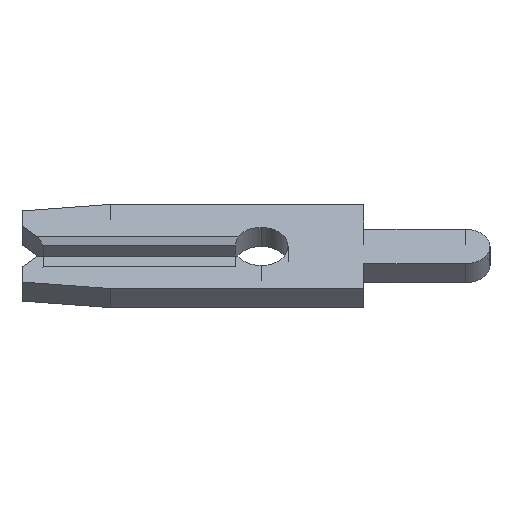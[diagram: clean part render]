
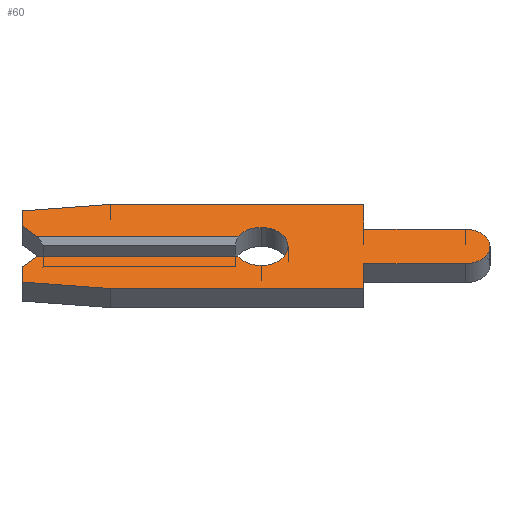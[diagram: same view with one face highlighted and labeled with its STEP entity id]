
A CAD part, left-side view. The second image highlights one B-rep face of the part: STEP entity #60.
In plain terms, the highlighted face is planar.
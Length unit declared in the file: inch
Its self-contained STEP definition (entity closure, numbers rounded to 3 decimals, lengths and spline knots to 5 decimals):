
#1 = LINE ( 'NONE', #1700, #1243 ) ;
#35 = DIRECTION ( 'NONE',  ( -1., 0., 0. ) ) ;
#55 = VECTOR ( 'NONE', #1398, 39.37008 ) ;
#60 = ADVANCED_FACE ( 'NONE', ( #71 ), #1540, .F. ) ;
#71 = FACE_OUTER_BOUND ( 'NONE', #1088, .T. ) ;
#76 = ORIENTED_EDGE ( 'NONE', *, *, #198, .F. ) ;
#86 = VECTOR ( 'NONE', #1055, 39.37008 ) ;
#87 = CARTESIAN_POINT ( 'NONE',  ( -0.013, -0.1975, -0.0235 ) ) ;
#91 = CARTESIAN_POINT ( 'NONE',  ( -0.013, -0.099, 0.0235 ) ) ;
#116 = EDGE_CURVE ( 'NONE', #1022, #850, #2049, .T. ) ;
#178 = VECTOR ( 'NONE', #1455, 39.37008 ) ;
#198 = EDGE_CURVE ( 'NONE', #300, #1527, #1787, .T. ) ;
#211 = ORIENTED_EDGE ( 'NONE', *, *, #1253, .F. ) ;
#213 = LINE ( 'NONE', #1473, #530 ) ;
#223 = VECTOR ( 'NONE', #612, 39.37008 ) ;
#226 = ORIENTED_EDGE ( 'NONE', *, *, #782, .F. ) ;
#241 = VECTOR ( 'NONE', #2071, 39.37008 ) ;
#256 = ORIENTED_EDGE ( 'NONE', *, *, #1232, .F. ) ;
#262 = CARTESIAN_POINT ( 'NONE',  ( -0.013, 0.146, -0.0575 ) ) ;
#300 = VERTEX_POINT ( 'NONE', #1580 ) ;
#330 = CARTESIAN_POINT ( 'NONE',  ( -0.013, 0.216, 0.013 ) ) ;
#331 = CARTESIAN_POINT ( 'NONE',  ( -0.013, -0.099, -0.0575 ) ) ;
#364 = DIRECTION ( 'NONE',  ( 0., 0., -1. ) ) ;
#389 = CARTESIAN_POINT ( 'NONE',  ( -0.013, 0.231, -0.028 ) ) ;
#399 = DIRECTION ( 'NONE',  ( 0., 0., -1. ) ) ;
#404 = ORIENTED_EDGE ( 'NONE', *, *, #1891, .F. ) ;
#419 = EDGE_CURVE ( 'NONE', #2013, #1078, #914, .T. ) ;
#432 = DIRECTION ( 'NONE',  ( 0., -1., 0. ) ) ;
#486 = ORIENTED_EDGE ( 'NONE', *, *, #760, .F. ) ;
#488 = ORIENTED_EDGE ( 'NONE', *, *, #1707, .F. ) ;
#492 = EDGE_CURVE ( 'NONE', #1858, #2013, #1421, .T. ) ;
#506 = LINE ( 'NONE', #1623, #223 ) ;
#515 = VERTEX_POINT ( 'NONE', #1100 ) ;
#530 = VECTOR ( 'NONE', #2150, 39.37008 ) ;
#537 = LINE ( 'NONE', #1904, #86 ) ;
#541 = ORIENTED_EDGE ( 'NONE', *, *, #1596, .F. ) ;
#547 = VERTEX_POINT ( 'NONE', #87 ) ;
#550 = VECTOR ( 'NONE', #1378, 39.37008 ) ;
#557 = VERTEX_POINT ( 'NONE', #590 ) ;
#568 = CARTESIAN_POINT ( 'NONE',  ( -0.013, 0.231, -0.04857 ) ) ;
#590 = CARTESIAN_POINT ( 'NONE',  ( -0.013, -0.099, 0.0235 ) ) ;
#593 = VERTEX_POINT ( 'NONE', #262 ) ;
#599 = CARTESIAN_POINT ( 'NONE',  ( -0.013, 0.146, 0.0575 ) ) ;
#612 = DIRECTION ( 'NONE',  ( 0., 1., 0. ) ) ;
#653 = DIRECTION ( 'NONE',  ( 1., 0., 0. ) ) ;
#684 = CARTESIAN_POINT ( 'NONE',  ( -0.013, 0.02252, 0.013 ) ) ;
#706 = DIRECTION ( 'NONE',  ( 1., 0., 0. ) ) ;
#720 = CARTESIAN_POINT ( 'NONE',  ( -0.013, -0.099, 0.0575 ) ) ;
#723 = LINE ( 'NONE', #1014, #1959 ) ;
#760 = EDGE_CURVE ( 'NONE', #1499, #2072, #213, .T. ) ;
#764 = CIRCLE ( 'NONE', #1404, 0.0235 ) ;
#771 = CARTESIAN_POINT ( 'NONE',  ( -0.013, 0., 0. ) ) ;
#782 = EDGE_CURVE ( 'NONE', #1078, #557, #1586, .T. ) ;
#793 = CIRCLE ( 'NONE', #1589, 0.026 ) ;
#801 = LINE ( 'NONE', #389, #1654 ) ;
#828 = DIRECTION ( 'NONE',  ( 0., 0.995, 0.105 ) ) ;
#840 = CARTESIAN_POINT ( 'NONE',  ( -0.013, 0.231, 0.028 ) ) ;
#844 = CARTESIAN_POINT ( 'NONE',  ( -0.013, 0.231, 0.04857 ) ) ;
#850 = VERTEX_POINT ( 'NONE', #1493 ) ;
#878 = DIRECTION ( 'NONE',  ( 0., 0., -1. ) ) ;
#879 = DIRECTION ( 'NONE',  ( 0., 1., 0. ) ) ;
#898 = DIRECTION ( 'NONE',  ( 0., 0., 1. ) ) ;
#910 = DIRECTION ( 'NONE',  ( 0., -1., 0. ) ) ;
#914 = LINE ( 'NONE', #599, #1304 ) ;
#919 = CARTESIAN_POINT ( 'NONE',  ( -0.013, 0., 0.026 ) ) ;
#953 = ORIENTED_EDGE ( 'NONE', *, *, #2076, .F. ) ;
#975 = EDGE_CURVE ( 'NONE', #515, #547, #764, .T. ) ;
#996 = CARTESIAN_POINT ( 'NONE',  ( -0.013, 0.02252, -0.013 ) ) ;
#1001 = EDGE_CURVE ( 'NONE', #2052, #300, #1039, .T. ) ;
#1014 = CARTESIAN_POINT ( 'NONE',  ( -0.013, 0.231, -0.04857 ) ) ;
#1022 = VERTEX_POINT ( 'NONE', #330 ) ;
#1039 = CIRCLE ( 'NONE', #1171, 0.026 ) ;
#1055 = DIRECTION ( 'NONE',  ( 0., -1., 0. ) ) ;
#1078 = VERTEX_POINT ( 'NONE', #2054 ) ;
#1088 = EDGE_LOOP ( 'NONE', ( #1475, #1601, #76, #2011, #2145, #211, #2048, #404, #953, #486, #488, #1652, #541, #226, #1982, #2135, #256, #1816 ) ) ;
#1100 = CARTESIAN_POINT ( 'NONE',  ( -0.013, -0.1975, 0.0235 ) ) ;
#1106 = LINE ( 'NONE', #1157, #1890 ) ;
#1121 = LINE ( 'NONE', #91, #1343 ) ;
#1136 = LINE ( 'NONE', #840, #55 ) ;
#1147 = CARTESIAN_POINT ( 'NONE',  ( -0.013, 0.231, -0.028 ) ) ;
#1157 = CARTESIAN_POINT ( 'NONE',  ( -0.013, 0.146, -0.0575 ) ) ;
#1164 = DIRECTION ( 'NONE',  ( 0., -1., 0. ) ) ;
#1171 = AXIS2_PLACEMENT_3D ( 'NONE', #2062, #35, #878 ) ;
#1186 = VERTEX_POINT ( 'NONE', #684 ) ;
#1196 = CARTESIAN_POINT ( 'NONE',  ( -0.013, 0.2105, 0.0075 ) ) ;
#1214 = DIRECTION ( 'NONE',  ( 0., -0.707, 0.707 ) ) ;
#1232 = EDGE_CURVE ( 'NONE', #850, #1858, #1136, .T. ) ;
#1243 = VECTOR ( 'NONE', #1164, 39.37008 ) ;
#1249 = EDGE_CURVE ( 'NONE', #1022, #1186, #537, .T. ) ;
#1253 = EDGE_CURVE ( 'NONE', #2036, #1752, #2004, .T. ) ;
#1271 = VECTOR ( 'NONE', #1214, 39.37008 ) ;
#1284 = VERTEX_POINT ( 'NONE', #568 ) ;
#1302 = CARTESIAN_POINT ( 'NONE',  ( -0.013, -0.1975, 0. ) ) ;
#1304 = VECTOR ( 'NONE', #432, 39.37008 ) ;
#1343 = VECTOR ( 'NONE', #910, 39.37008 ) ;
#1378 = DIRECTION ( 'NONE',  ( 0., 0.707, 0.707 ) ) ;
#1398 = DIRECTION ( 'NONE',  ( 0., 0., 1. ) ) ;
#1404 = AXIS2_PLACEMENT_3D ( 'NONE', #1302, #653, #1829 ) ;
#1421 = LINE ( 'NONE', #1772, #178 ) ;
#1455 = DIRECTION ( 'NONE',  ( 0., -0.995, 0.105 ) ) ;
#1473 = CARTESIAN_POINT ( 'NONE',  ( -0.013, -0.099, -0.0575 ) ) ;
#1475 = ORIENTED_EDGE ( 'NONE', *, *, #1249, .T. ) ;
#1493 = CARTESIAN_POINT ( 'NONE',  ( -0.013, 0.231, 0.028 ) ) ;
#1499 = VERTEX_POINT ( 'NONE', #1774 ) ;
#1527 = VERTEX_POINT ( 'NONE', #919 ) ;
#1540 = PLANE ( 'NONE',  #1711 ) ;
#1569 = CARTESIAN_POINT ( 'NONE',  ( -0.013, 0., 0. ) ) ;
#1580 = CARTESIAN_POINT ( 'NONE',  ( -0.013, 0., -0.026 ) ) ;
#1584 = EDGE_CURVE ( 'NONE', #1527, #1186, #793, .T. ) ;
#1586 = LINE ( 'NONE', #720, #241 ) ;
#1589 = AXIS2_PLACEMENT_3D ( 'NONE', #771, #2115, #399 ) ;
#1596 = EDGE_CURVE ( 'NONE', #557, #515, #1121, .T. ) ;
#1601 = ORIENTED_EDGE ( 'NONE', *, *, #1584, .F. ) ;
#1623 = CARTESIAN_POINT ( 'NONE',  ( -0.013, -0.099, -0.0235 ) ) ;
#1652 = ORIENTED_EDGE ( 'NONE', *, *, #975, .F. ) ;
#1654 = VECTOR ( 'NONE', #898, 39.37008 ) ;
#1686 = EDGE_CURVE ( 'NONE', #1284, #2036, #801, .T. ) ;
#1693 = CARTESIAN_POINT ( 'NONE',  ( -0.013, 0.146, 0.0575 ) ) ;
#1700 = CARTESIAN_POINT ( 'NONE',  ( -0.013, 0., -0.013 ) ) ;
#1707 = EDGE_CURVE ( 'NONE', #547, #1499, #506, .T. ) ;
#1711 = AXIS2_PLACEMENT_3D ( 'NONE', #1569, #706, #364 ) ;
#1730 = DIRECTION ( 'NONE',  ( 0., 0., -1. ) ) ;
#1752 = VERTEX_POINT ( 'NONE', #1783 ) ;
#1772 = CARTESIAN_POINT ( 'NONE',  ( -0.013, 0.231, 0.04857 ) ) ;
#1774 = CARTESIAN_POINT ( 'NONE',  ( -0.013, -0.099, -0.0235 ) ) ;
#1783 = CARTESIAN_POINT ( 'NONE',  ( -0.013, 0.216, -0.013 ) ) ;
#1787 = CIRCLE ( 'NONE', #2043, 0.026 ) ;
#1816 = ORIENTED_EDGE ( 'NONE', *, *, #116, .F. ) ;
#1829 = DIRECTION ( 'NONE',  ( 0., 0., 1. ) ) ;
#1847 = EDGE_CURVE ( 'NONE', #1752, #2052, #1, .T. ) ;
#1858 = VERTEX_POINT ( 'NONE', #844 ) ;
#1868 = CARTESIAN_POINT ( 'NONE',  ( -0.013, 0.2105, -0.0075 ) ) ;
#1890 = VECTOR ( 'NONE', #879, 39.37008 ) ;
#1891 = EDGE_CURVE ( 'NONE', #593, #1284, #723, .T. ) ;
#1902 = DIRECTION ( 'NONE',  ( -1., 0., 0. ) ) ;
#1904 = CARTESIAN_POINT ( 'NONE',  ( -0.013, 0.231, 0.013 ) ) ;
#1959 = VECTOR ( 'NONE', #828, 39.37008 ) ;
#1982 = ORIENTED_EDGE ( 'NONE', *, *, #419, .F. ) ;
#2004 = LINE ( 'NONE', #1868, #1271 ) ;
#2011 = ORIENTED_EDGE ( 'NONE', *, *, #1001, .F. ) ;
#2013 = VERTEX_POINT ( 'NONE', #1693 ) ;
#2036 = VERTEX_POINT ( 'NONE', #1147 ) ;
#2043 = AXIS2_PLACEMENT_3D ( 'NONE', #2081, #1902, #1730 ) ;
#2048 = ORIENTED_EDGE ( 'NONE', *, *, #1686, .F. ) ;
#2049 = LINE ( 'NONE', #1196, #550 ) ;
#2052 = VERTEX_POINT ( 'NONE', #996 ) ;
#2054 = CARTESIAN_POINT ( 'NONE',  ( -0.013, -0.099, 0.0575 ) ) ;
#2062 = CARTESIAN_POINT ( 'NONE',  ( -0.013, 0., 0. ) ) ;
#2071 = DIRECTION ( 'NONE',  ( 0., 0., -1. ) ) ;
#2072 = VERTEX_POINT ( 'NONE', #331 ) ;
#2076 = EDGE_CURVE ( 'NONE', #2072, #593, #1106, .T. ) ;
#2081 = CARTESIAN_POINT ( 'NONE',  ( -0.013, 0., 0. ) ) ;
#2115 = DIRECTION ( 'NONE',  ( -1., 0., 0. ) ) ;
#2135 = ORIENTED_EDGE ( 'NONE', *, *, #492, .F. ) ;
#2145 = ORIENTED_EDGE ( 'NONE', *, *, #1847, .F. ) ;
#2150 = DIRECTION ( 'NONE',  ( 0., 0., -1. ) ) ;
